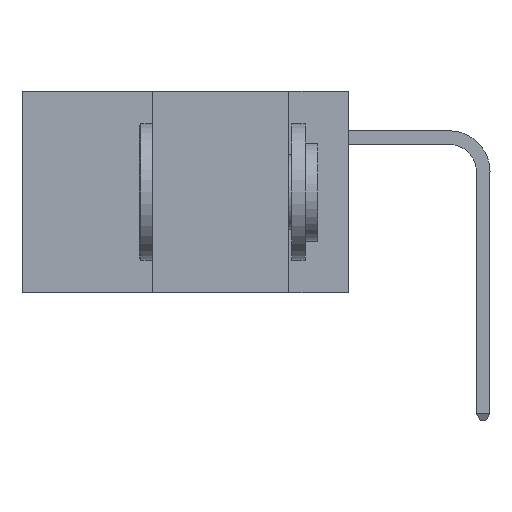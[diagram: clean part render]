
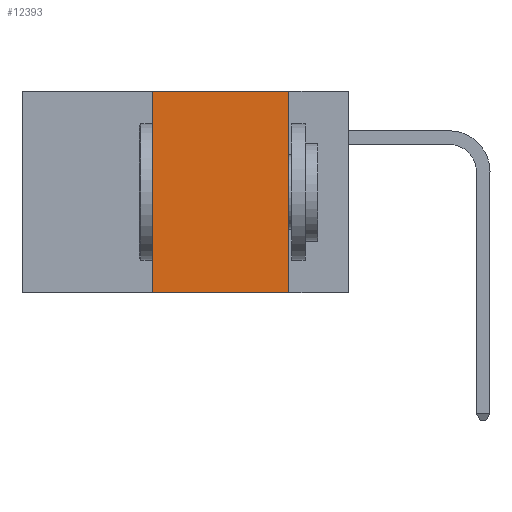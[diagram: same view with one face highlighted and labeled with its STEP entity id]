
A CAD part, left-side view. The second image highlights one B-rep face of the part: STEP entity #12393.
In plain terms, the highlighted planar face has unit normal (-1, 0, 0).
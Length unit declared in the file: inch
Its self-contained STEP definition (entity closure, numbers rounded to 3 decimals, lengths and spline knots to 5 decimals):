
#29 = EDGE_CURVE ( 'NONE', #5518, #17494, #18003, .T. ) ;
#116 = FACE_OUTER_BOUND ( 'NONE', #3758, .T. ) ;
#343 = DIRECTION ( 'NONE',  ( 0., 0., -1. ) ) ;
#463 = CARTESIAN_POINT ( 'NONE',  ( 0., 0.6, 0. ) ) ;
#912 = DIRECTION ( 'NONE',  ( 0., 0., 1. ) ) ;
#1536 = DIRECTION ( 'NONE',  ( 0., -1., 0. ) ) ;
#2315 = VERTEX_POINT ( 'NONE', #7518 ) ;
#2378 = ORIENTED_EDGE ( 'NONE', *, *, #29, .T. ) ;
#3275 = EDGE_CURVE ( 'NONE', #5518, #2315, #13408, .T. ) ;
#3758 = EDGE_LOOP ( 'NONE', ( #7534, #9309, #17068, #2378 ) ) ;
#4768 = CARTESIAN_POINT ( 'NONE',  ( 0., 0.6, 0. ) ) ;
#4935 = DIRECTION ( 'NONE',  ( 0., -1., 0. ) ) ;
#5518 = VERTEX_POINT ( 'NONE', #7339 ) ;
#5814 = VECTOR ( 'NONE', #4935, 39.37008 ) ;
#5985 = VECTOR ( 'NONE', #912, 39.37008 ) ;
#6781 = VECTOR ( 'NONE', #7042, 39.37008 ) ;
#7042 = DIRECTION ( 'NONE',  ( 0., 0., -1. ) ) ;
#7062 = AXIS2_PLACEMENT_3D ( 'NONE', #4768, #8994, #343 ) ;
#7339 = CARTESIAN_POINT ( 'NONE',  ( 0., 0.36, -0.37 ) ) ;
#7399 = VECTOR ( 'NONE', #1536, 39.37008 ) ;
#7518 = CARTESIAN_POINT ( 'NONE',  ( 0., 0.36, 0. ) ) ;
#7534 = ORIENTED_EDGE ( 'NONE', *, *, #17084, .F. ) ;
#7562 = PLANE ( 'NONE',  #7062 ) ;
#8742 = VERTEX_POINT ( 'NONE', #16444 ) ;
#8994 = DIRECTION ( 'NONE',  ( 1., 0., 0. ) ) ;
#9309 = ORIENTED_EDGE ( 'NONE', *, *, #14983, .F. ) ;
#9584 = CARTESIAN_POINT ( 'NONE',  ( 0., 0.11, -0.37 ) ) ;
#10226 = CARTESIAN_POINT ( 'NONE',  ( 0., 0.6, -0.37 ) ) ;
#10549 = LINE ( 'NONE', #16742, #6781 ) ;
#10935 = CARTESIAN_POINT ( 'NONE',  ( 0., 0.36, 0. ) ) ;
#12393 = ADVANCED_FACE ( 'NONE', ( #116 ), #7562, .F. ) ;
#13408 = LINE ( 'NONE', #10935, #5985 ) ;
#14983 = EDGE_CURVE ( 'NONE', #2315, #8742, #17702, .T. ) ;
#16444 = CARTESIAN_POINT ( 'NONE',  ( 0., 0.11, 0. ) ) ;
#16742 = CARTESIAN_POINT ( 'NONE',  ( 0., 0.11, 0. ) ) ;
#17068 = ORIENTED_EDGE ( 'NONE', *, *, #3275, .F. ) ;
#17084 = EDGE_CURVE ( 'NONE', #8742, #17494, #10549, .T. ) ;
#17494 = VERTEX_POINT ( 'NONE', #9584 ) ;
#17702 = LINE ( 'NONE', #463, #5814 ) ;
#18003 = LINE ( 'NONE', #10226, #7399 ) ;
